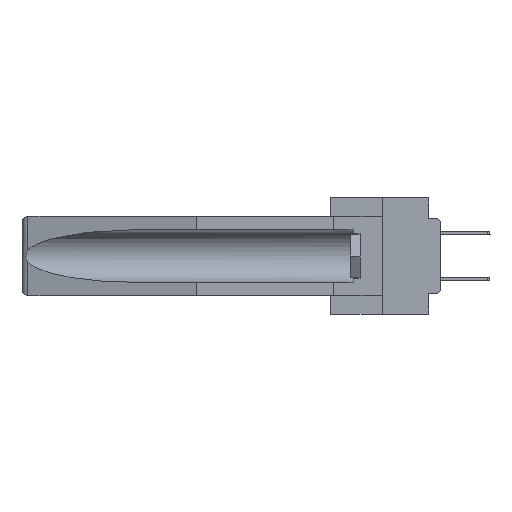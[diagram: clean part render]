
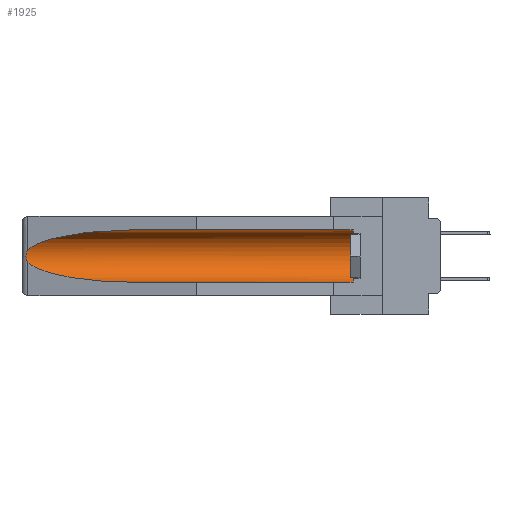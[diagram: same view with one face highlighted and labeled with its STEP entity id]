
A CAD part, left-side view. The second image highlights one B-rep face of the part: STEP entity #1925.
In plain terms, the highlighted cylindrical face has radius 2.857 mm (diameter 5.715 mm), a partial arc.
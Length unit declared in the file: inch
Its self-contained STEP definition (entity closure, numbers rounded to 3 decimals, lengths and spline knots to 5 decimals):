
#400 = EDGE_CURVE ( 'NONE', #10182, #31726, #27909, .T. ) ;
#1173 = CARTESIAN_POINT ( 'NONE',  ( 0.26537, 1.52718, -0.19328 ) ) ;
#1590 = EDGE_CURVE ( 'NONE', #1761, #31726, #19332, .T. ) ;
#1670 = CARTESIAN_POINT ( 'NONE',  ( 0.26537, 1.52718, -0.19328 ) ) ;
#1761 = VERTEX_POINT ( 'NONE', #31296 ) ;
#1870 = ORIENTED_EDGE ( 'NONE', *, *, #1590, .T. ) ;
#1925 = ADVANCED_FACE ( 'NONE', ( #26695 ), #29238, .F. ) ;
#2391 = CIRCLE ( 'NONE', #15970, 0.1125 ) ;
#2534 = EDGE_LOOP ( 'NONE', ( #25019, #5445, #1870, #2962, #15230, #18592 ) ) ;
#2962 = ORIENTED_EDGE ( 'NONE', *, *, #400, .F. ) ;
#3328 = CARTESIAN_POINT ( 'NONE',  ( 0.155, 0.126, -0.284 ) ) ;
#4327 = DIRECTION ( 'NONE',  ( 0., 0., 1. ) ) ;
#4510 = VERTEX_POINT ( 'NONE', #20904 ) ;
#4531 = LINE ( 'NONE', #5020, #25566 ) ;
#5020 = CARTESIAN_POINT ( 'NONE',  ( 0.155, -0.30754, -0.059 ) ) ;
#5445 = ORIENTED_EDGE ( 'NONE', *, *, #27284, .T. ) ;
#5767 = CARTESIAN_POINT ( 'NONE',  ( 0.155, -0.30754, -0.1715 ) ) ;
#5794 = CARTESIAN_POINT ( 'NONE',  ( 0.25451, 1.48313, -0.09465 ) ) ;
#6617 = EDGE_CURVE ( 'NONE', #26914, #4510, #4531, .T. ) ;
#6963 = CARTESIAN_POINT ( 'NONE',  ( 0.2675, 1.53308, -0.16763 ) ) ;
#7187 = CARTESIAN_POINT ( 'NONE',  ( 0.155, 1.07973, -0.284 ) ) ;
#10182 = VERTEX_POINT ( 'NONE', #3328 ) ;
#11392 = CARTESIAN_POINT ( 'NONE',  ( 0.26537, 1.52718, -0.14972 ) ) ;
#11590 = CARTESIAN_POINT ( 'NONE',  ( 0.155, 0.126, -0.059 ) ) ;
#11817 = DIRECTION ( 'NONE',  ( 0., -1., 0. ) ) ;
#11895 = CARTESIAN_POINT ( 'NONE',  ( 0.2673, 1.53269, -0.17917 ) ) ;
#13111 = CARTESIAN_POINT ( 'NONE',  ( 0.21114, 1.30732, -0.059 ) ) ;
#13761 = DIRECTION ( 'NONE',  ( 0., 0., 1. ) ) ;
#15042 = CARTESIAN_POINT ( 'NONE',  ( 0.26537, 1.52718, -0.14972 ) ) ;
#15207 = AXIS2_PLACEMENT_3D ( 'NONE', #5767, #16136, #13761 ) ;
#15230 = ORIENTED_EDGE ( 'NONE', *, *, #17343, .T. ) ;
#15970 = AXIS2_PLACEMENT_3D ( 'NONE', #17575, #11817, #4327 ) ;
#16136 = DIRECTION ( 'NONE',  ( 0., 1., 0. ) ) ;
#16172 = CARTESIAN_POINT ( 'NONE',  ( 0.26537, 1.52718, -0.14972 ) ) ;
#17151 = CARTESIAN_POINT ( 'NONE',  ( 0.26597, 1.52961, -0.15275 ) ) ;
#17343 = EDGE_CURVE ( 'NONE', #10182, #26914, #2391, .T. ) ;
#17398 = VERTEX_POINT ( 'NONE', #15042 ) ;
#17575 = CARTESIAN_POINT ( 'NONE',  ( 0.155, 0.126, -0.1715 ) ) ;
#18592 = ORIENTED_EDGE ( 'NONE', *, *, #6617, .T. ) ;
#19332 =( BOUNDED_CURVE ( )  B_SPLINE_CURVE ( 3, ( #1173, #29115, #21940, #32335 ),
 .UNSPECIFIED., .F., .F. ) 
 B_SPLINE_CURVE_WITH_KNOTS ( ( 4, 4 ),
 ( 0.1948, 1.5708 ),
 .UNSPECIFIED. ) 
 CURVE ( )  GEOMETRIC_REPRESENTATION_ITEM ( )  RATIONAL_B_SPLINE_CURVE ( ( 1., 0.848, 0.848, 1. ) ) 
 REPRESENTATION_ITEM ( '' )  );
#19372 = CARTESIAN_POINT ( 'NONE',  ( 0.2673, 1.5327, -0.16383 ) ) ;
#20904 = CARTESIAN_POINT ( 'NONE',  ( 0.155, 1.07973, -0.059 ) ) ;
#21940 = CARTESIAN_POINT ( 'NONE',  ( 0.21114, 1.30732, -0.284 ) ) ;
#22262 = CARTESIAN_POINT ( 'NONE',  ( 0.26597, 1.5296, -0.19026 ) ) ;
#22279 = CARTESIAN_POINT ( 'NONE',  ( 0.155, -0.30754, -0.284 ) ) ;
#23465 = CARTESIAN_POINT ( 'NONE',  ( 0.155, 1.07973, -0.059 ) ) ;
#24476 = CARTESIAN_POINT ( 'NONE',  ( 0.2675, 1.53308, -0.17534 ) ) ;
#24985 = CARTESIAN_POINT ( 'NONE',  ( 0.26655, 1.53094, -0.18657 ) ) ;
#25019 = ORIENTED_EDGE ( 'NONE', *, *, #31908, .T. ) ;
#25566 = VECTOR ( 'NONE', #27677, 39.37008 ) ;
#26695 = FACE_OUTER_BOUND ( 'NONE', #2534, .T. ) ;
#26914 = VERTEX_POINT ( 'NONE', #11590 ) ;
#27038 = CARTESIAN_POINT ( 'NONE',  ( 0.26654, 1.53092, -0.15636 ) ) ;
#27284 = EDGE_CURVE ( 'NONE', #17398, #1761, #27482, .T. ) ;
#27482 = B_SPLINE_CURVE_WITH_KNOTS ( 'NONE', 3,
 ( #11392, #17151, #27038, #19372, #6963, #24476, #11895, #24985, #22262, #1670 ),
 .UNSPECIFIED., .F., .F.,
 ( 4, 2, 2, 2, 4 ),
 ( 0., 0.00029, 0.00058, 0.00087, 0.00117 ),
 .UNSPECIFIED. ) ;
#27677 = DIRECTION ( 'NONE',  ( 0., 1., 0. ) ) ;
#27909 = LINE ( 'NONE', #22279, #29710 ) ;
#29115 = CARTESIAN_POINT ( 'NONE',  ( 0.25451, 1.48313, -0.24835 ) ) ;
#29238 = CYLINDRICAL_SURFACE ( 'NONE', #15207, 0.1125 ) ;
#29710 = VECTOR ( 'NONE', #32667, 39.37008 ) ;
#31296 = CARTESIAN_POINT ( 'NONE',  ( 0.26537, 1.52718, -0.19328 ) ) ;
#31726 = VERTEX_POINT ( 'NONE', #7187 ) ;
#31908 = EDGE_CURVE ( 'NONE', #4510, #17398, #33054, .T. ) ;
#32335 = CARTESIAN_POINT ( 'NONE',  ( 0.155, 1.07973, -0.284 ) ) ;
#32667 = DIRECTION ( 'NONE',  ( 0., 1., 0. ) ) ;
#33054 =( BOUNDED_CURVE ( )  B_SPLINE_CURVE ( 3, ( #23465, #13111, #5794, #16172 ),
 .UNSPECIFIED., .F., .F. ) 
 B_SPLINE_CURVE_WITH_KNOTS ( ( 4, 4 ),
 ( 4.71239, 6.08839 ),
 .UNSPECIFIED. ) 
 CURVE ( )  GEOMETRIC_REPRESENTATION_ITEM ( )  RATIONAL_B_SPLINE_CURVE ( ( 1., 0.848, 0.848, 1. ) ) 
 REPRESENTATION_ITEM ( '' )  );
